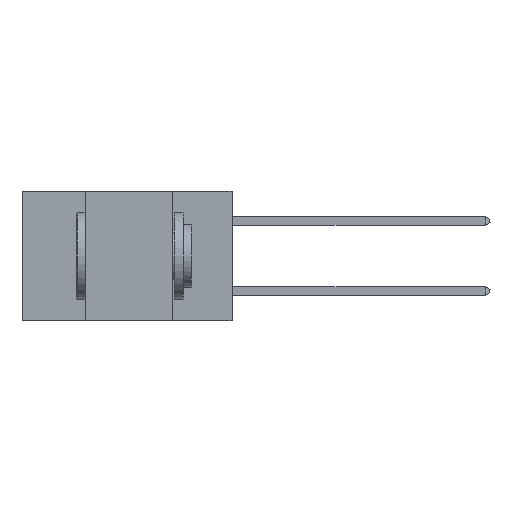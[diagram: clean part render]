
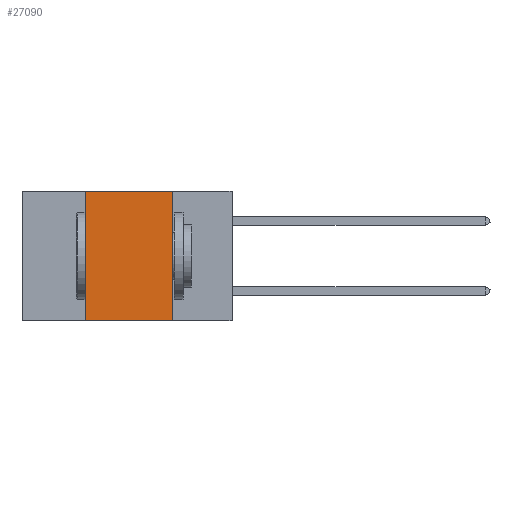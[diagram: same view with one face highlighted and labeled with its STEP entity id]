
A CAD part, left-side view. The second image highlights one B-rep face of the part: STEP entity #27090.
In plain terms, the highlighted planar face has unit normal (-1, 0, 0).
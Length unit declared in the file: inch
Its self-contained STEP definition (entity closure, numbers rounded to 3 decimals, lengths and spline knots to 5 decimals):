
#11 = CARTESIAN_POINT ( 'NONE',  ( 0., 0.17, 0. ) ) ;
#825 = DIRECTION ( 'NONE',  ( 0., 0., -1. ) ) ;
#3630 = ORIENTED_EDGE ( 'NONE', *, *, #19091, .F. ) ;
#4250 = DIRECTION ( 'NONE',  ( 0., 0., 1. ) ) ;
#4334 = ORIENTED_EDGE ( 'NONE', *, *, #8802, .F. ) ;
#4709 = VECTOR ( 'NONE', #6803, 39.37008 ) ;
#4715 = VECTOR ( 'NONE', #11516, 39.37008 ) ;
#5742 = AXIS2_PLACEMENT_3D ( 'NONE', #13457, #9076, #24392 ) ;
#6220 = VECTOR ( 'NONE', #825, 39.37008 ) ;
#6803 = DIRECTION ( 'NONE',  ( 0., -1., 0. ) ) ;
#8802 = EDGE_CURVE ( 'NONE', #13432, #18158, #16465, .T. ) ;
#9076 = DIRECTION ( 'NONE',  ( 1., 0., 0. ) ) ;
#9661 = CARTESIAN_POINT ( 'NONE',  ( 0., 0.17, 0. ) ) ;
#9786 = CARTESIAN_POINT ( 'NONE',  ( 0., 0.42, 0. ) ) ;
#9949 = VECTOR ( 'NONE', #4250, 39.37008 ) ;
#10225 = ORIENTED_EDGE ( 'NONE', *, *, #13794, .F. ) ;
#11516 = DIRECTION ( 'NONE',  ( 0., -1., 0. ) ) ;
#12096 = LINE ( 'NONE', #9661, #6220 ) ;
#13432 = VERTEX_POINT ( 'NONE', #9786 ) ;
#13457 = CARTESIAN_POINT ( 'NONE',  ( 0., 0.6, 0. ) ) ;
#13794 = EDGE_CURVE ( 'NONE', #22780, #13432, #21653, .T. ) ;
#14620 = EDGE_CURVE ( 'NONE', #22780, #19424, #17182, .T. ) ;
#16465 = LINE ( 'NONE', #17814, #4709 ) ;
#17182 = LINE ( 'NONE', #26696, #4715 ) ;
#17814 = CARTESIAN_POINT ( 'NONE',  ( 0., 0.6, 0. ) ) ;
#17884 = PLANE ( 'NONE',  #5742 ) ;
#18158 = VERTEX_POINT ( 'NONE', #11 ) ;
#19091 = EDGE_CURVE ( 'NONE', #18158, #19424, #12096, .T. ) ;
#19424 = VERTEX_POINT ( 'NONE', #28114 ) ;
#19719 = CARTESIAN_POINT ( 'NONE',  ( 0., 0.42, 0. ) ) ;
#20450 = FACE_OUTER_BOUND ( 'NONE', #20768, .T. ) ;
#20768 = EDGE_LOOP ( 'NONE', ( #3630, #4334, #10225, #21912 ) ) ;
#21653 = LINE ( 'NONE', #19719, #9949 ) ;
#21912 = ORIENTED_EDGE ( 'NONE', *, *, #14620, .T. ) ;
#22780 = VERTEX_POINT ( 'NONE', #26431 ) ;
#24392 = DIRECTION ( 'NONE',  ( 0., 0., -1. ) ) ;
#26431 = CARTESIAN_POINT ( 'NONE',  ( 0., 0.42, -0.37 ) ) ;
#26696 = CARTESIAN_POINT ( 'NONE',  ( 0., 0.6, -0.37 ) ) ;
#27090 = ADVANCED_FACE ( 'NONE', ( #20450 ), #17884, .F. ) ;
#28114 = CARTESIAN_POINT ( 'NONE',  ( 0., 0.17, -0.37 ) ) ;
